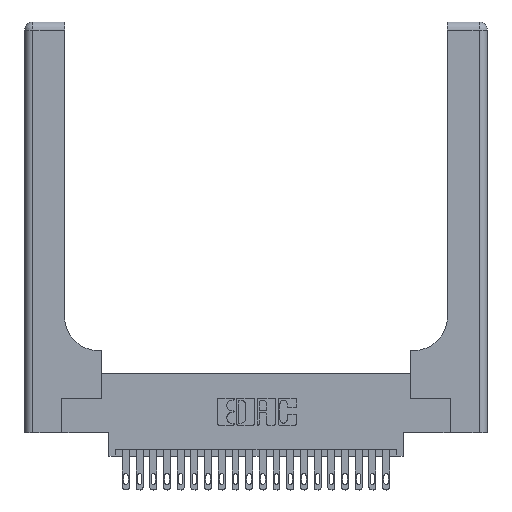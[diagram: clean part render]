
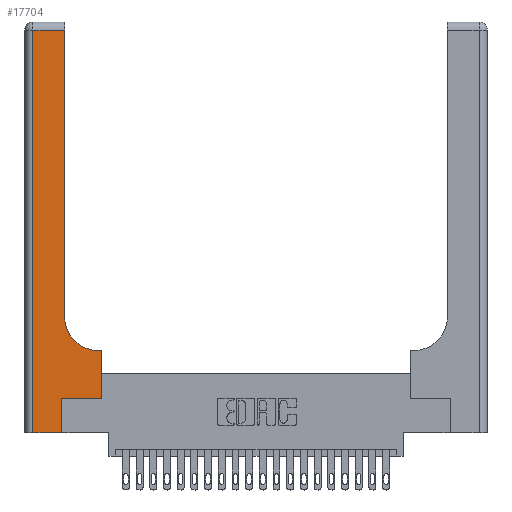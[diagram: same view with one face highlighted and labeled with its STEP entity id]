
A CAD part, top view. The second image highlights one B-rep face of the part: STEP entity #17704.
In plain terms, the highlighted planar face has unit normal (0, 0, 1).
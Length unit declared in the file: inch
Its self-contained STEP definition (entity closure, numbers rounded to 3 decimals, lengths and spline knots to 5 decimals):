
#535 = DIRECTION ( 'NONE',  ( 1., 0., 0. ) ) ;
#1446 = VECTOR ( 'NONE', #8071, 39.37008 ) ;
#1471 = EDGE_LOOP ( 'NONE', ( #14289, #21490, #14722, #1939, #2243, #16055, #1617, #23156, #17588 ) ) ;
#1617 = ORIENTED_EDGE ( 'NONE', *, *, #19934, .T. ) ;
#1696 = CARTESIAN_POINT ( 'NONE',  ( 0.2915, 0.6, 0.37 ) ) ;
#1939 = ORIENTED_EDGE ( 'NONE', *, *, #8741, .T. ) ;
#2243 = ORIENTED_EDGE ( 'NONE', *, *, #20885, .T. ) ;
#2472 = DIRECTION ( 'NONE',  ( 0., 0., -1. ) ) ;
#2663 = CARTESIAN_POINT ( 'NONE',  ( 0., 2.94, 0.37 ) ) ;
#2815 = DIRECTION ( 'NONE',  ( 0., 1., 0. ) ) ;
#2955 = CARTESIAN_POINT ( 'NONE',  ( 0.269, 0., 0.37 ) ) ;
#3945 = CARTESIAN_POINT ( 'NONE',  ( 0.269, 0.25, 0.37 ) ) ;
#3994 = CARTESIAN_POINT ( 'NONE',  ( 0.5585, 0.6, 0.37 ) ) ;
#4305 = DIRECTION ( 'NONE',  ( -1., 0., 0. ) ) ;
#4435 = CARTESIAN_POINT ( 'NONE',  ( 0.2915, 0.85, 0.37 ) ) ;
#5079 = LINE ( 'NONE', #2955, #22720 ) ;
#5213 = DIRECTION ( 'NONE',  ( 1., 0., 0. ) ) ;
#5769 = CARTESIAN_POINT ( 'NONE',  ( 0.269, 0., 0.37 ) ) ;
#5780 = VERTEX_POINT ( 'NONE', #3994 ) ;
#5906 = CARTESIAN_POINT ( 'NONE',  ( 0., 3., 0.37 ) ) ;
#5979 = CARTESIAN_POINT ( 'NONE',  ( 0.06, 2.94, 0.37 ) ) ;
#6341 = VECTOR ( 'NONE', #11238, 39.37008 ) ;
#7574 = VERTEX_POINT ( 'NONE', #23686 ) ;
#7920 = CARTESIAN_POINT ( 'NONE',  ( 0.5585, 0.25, 0.37 ) ) ;
#8071 = DIRECTION ( 'NONE',  ( -1., 0., 0. ) ) ;
#8370 = CARTESIAN_POINT ( 'NONE',  ( 0.5585, 0.25, 0.37 ) ) ;
#8741 = EDGE_CURVE ( 'NONE', #18857, #19370, #15092, .T. ) ;
#9144 = CIRCLE ( 'NONE', #18328, 0.25 ) ;
#9267 = EDGE_CURVE ( 'NONE', #9975, #7574, #12441, .T. ) ;
#9906 = EDGE_CURVE ( 'NONE', #15528, #18857, #17949, .T. ) ;
#9975 = VERTEX_POINT ( 'NONE', #4435 ) ;
#10541 = CARTESIAN_POINT ( 'NONE',  ( 0., 0., 0.37 ) ) ;
#10740 = DIRECTION ( 'NONE',  ( 0., -1., 0. ) ) ;
#11063 = CARTESIAN_POINT ( 'NONE',  ( 0.5415, 0.6, 0.37 ) ) ;
#11238 = DIRECTION ( 'NONE',  ( 1., 0., 0. ) ) ;
#11270 = EDGE_CURVE ( 'NONE', #7574, #15528, #20479, .T. ) ;
#11643 = AXIS2_PLACEMENT_3D ( 'NONE', #5906, #11713, #4305 ) ;
#11713 = DIRECTION ( 'NONE',  ( 0., 0., -1. ) ) ;
#11978 = CARTESIAN_POINT ( 'NONE',  ( 0.06, 0., 0.37 ) ) ;
#12441 = LINE ( 'NONE', #19479, #14203 ) ;
#12731 = LINE ( 'NONE', #3945, #6341 ) ;
#13748 = DIRECTION ( 'NONE',  ( 0., 1., 0. ) ) ;
#14203 = VECTOR ( 'NONE', #13748, 39.37008 ) ;
#14289 = ORIENTED_EDGE ( 'NONE', *, *, #9267, .T. ) ;
#14315 = EDGE_CURVE ( 'NONE', #18047, #9975, #9144, .T. ) ;
#14498 = VERTEX_POINT ( 'NONE', #8370 ) ;
#14722 = ORIENTED_EDGE ( 'NONE', *, *, #9906, .T. ) ;
#15006 = VERTEX_POINT ( 'NONE', #17320 ) ;
#15092 = LINE ( 'NONE', #10541, #20877 ) ;
#15528 = VERTEX_POINT ( 'NONE', #5979 ) ;
#16055 = ORIENTED_EDGE ( 'NONE', *, *, #17593, .T. ) ;
#16450 = VECTOR ( 'NONE', #22688, 39.37008 ) ;
#17320 = CARTESIAN_POINT ( 'NONE',  ( 0.269, 0.25, 0.37 ) ) ;
#17588 = ORIENTED_EDGE ( 'NONE', *, *, #14315, .T. ) ;
#17593 = EDGE_CURVE ( 'NONE', #15006, #14498, #12731, .T. ) ;
#17704 = ADVANCED_FACE ( 'NONE', ( #20818 ), #19151, .F. ) ;
#17949 = LINE ( 'NONE', #23814, #20548 ) ;
#18046 = DIRECTION ( 'NONE',  ( -1., 0., 0. ) ) ;
#18047 = VERTEX_POINT ( 'NONE', #11063 ) ;
#18328 = AXIS2_PLACEMENT_3D ( 'NONE', #18997, #2472, #535 ) ;
#18857 = VERTEX_POINT ( 'NONE', #11978 ) ;
#18997 = CARTESIAN_POINT ( 'NONE',  ( 0.5415, 0.85, 0.37 ) ) ;
#19151 = PLANE ( 'NONE',  #11643 ) ;
#19370 = VERTEX_POINT ( 'NONE', #5769 ) ;
#19479 = CARTESIAN_POINT ( 'NONE',  ( 0.2915, 3., 0.37 ) ) ;
#19689 = LINE ( 'NONE', #1696, #22899 ) ;
#19934 = EDGE_CURVE ( 'NONE', #14498, #5780, #22812, .T. ) ;
#20479 = LINE ( 'NONE', #2663, #1446 ) ;
#20548 = VECTOR ( 'NONE', #10740, 39.37008 ) ;
#20818 = FACE_OUTER_BOUND ( 'NONE', #1471, .T. ) ;
#20877 = VECTOR ( 'NONE', #5213, 39.37008 ) ;
#20885 = EDGE_CURVE ( 'NONE', #19370, #15006, #5079, .T. ) ;
#21490 = ORIENTED_EDGE ( 'NONE', *, *, #11270, .T. ) ;
#22688 = DIRECTION ( 'NONE',  ( 0., 1., 0. ) ) ;
#22720 = VECTOR ( 'NONE', #2815, 39.37008 ) ;
#22812 = LINE ( 'NONE', #7920, #16450 ) ;
#22899 = VECTOR ( 'NONE', #18046, 39.37008 ) ;
#23156 = ORIENTED_EDGE ( 'NONE', *, *, #23656, .T. ) ;
#23656 = EDGE_CURVE ( 'NONE', #5780, #18047, #19689, .T. ) ;
#23686 = CARTESIAN_POINT ( 'NONE',  ( 0.2915, 2.94, 0.37 ) ) ;
#23814 = CARTESIAN_POINT ( 'NONE',  ( 0.06, 3., 0.37 ) ) ;
